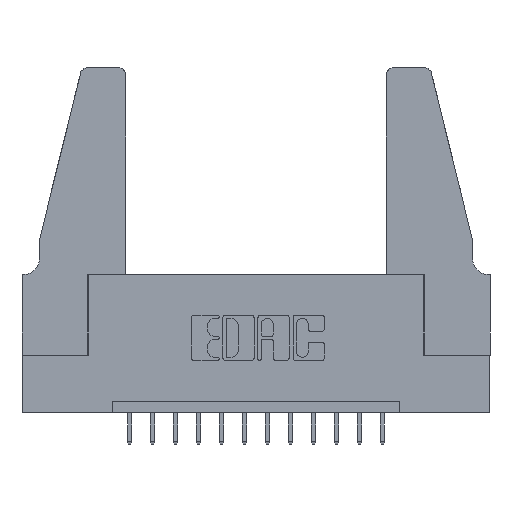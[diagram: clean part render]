
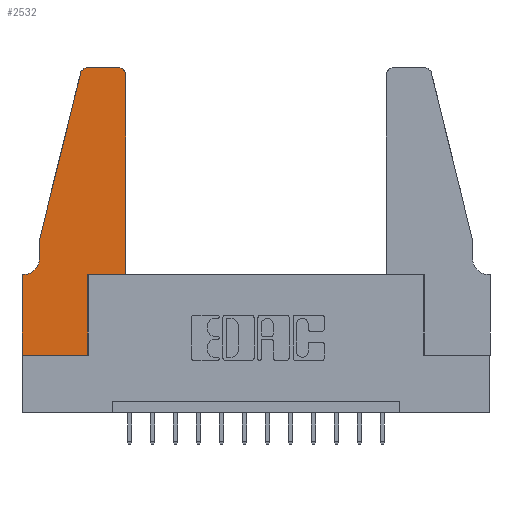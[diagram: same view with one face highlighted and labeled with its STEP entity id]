
A CAD part, top view. The second image highlights one B-rep face of the part: STEP entity #2532.
In plain terms, the highlighted planar face has unit normal (0, 0, 1).
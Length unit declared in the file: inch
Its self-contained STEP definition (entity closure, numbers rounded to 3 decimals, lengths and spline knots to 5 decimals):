
#18 = CIRCLE ( 'NONE', #11860, 0.03 ) ;
#235 = CARTESIAN_POINT ( 'NONE',  ( 0.4505, 0.35, 0.37 ) ) ;
#239 = EDGE_CURVE ( 'NONE', #14840, #13316, #10467, .T. ) ;
#318 = VERTEX_POINT ( 'NONE', #13299 ) ;
#398 = DIRECTION ( 'NONE',  ( 0., 1., 0. ) ) ;
#469 = DIRECTION ( 'NONE',  ( 0., 0., 1. ) ) ;
#522 = CARTESIAN_POINT ( 'NONE',  ( 0.0055, 0.35, 0.37 ) ) ;
#626 = VECTOR ( 'NONE', #9659, 39.37008 ) ;
#684 = CARTESIAN_POINT ( 'NONE',  ( 0.0755, 0.35, 0.37 ) ) ;
#812 = CARTESIAN_POINT ( 'NONE',  ( 0., 0., 0.37 ) ) ;
#1012 = AXIS2_PLACEMENT_3D ( 'NONE', #2104, #15271, #14018 ) ;
#1308 = PLANE ( 'NONE',  #6157 ) ;
#1349 = ORIENTED_EDGE ( 'NONE', *, *, #14159, .T. ) ;
#1703 = CARTESIAN_POINT ( 'NONE',  ( 0.4505, 0.35, 0.37 ) ) ;
#1771 = DIRECTION ( 'NONE',  ( -1., 0., 0. ) ) ;
#1816 = EDGE_CURVE ( 'NONE', #4853, #5259, #2169, .T. ) ;
#2104 = CARTESIAN_POINT ( 'NONE',  ( 0.0055, 0.42, 0.37 ) ) ;
#2169 = CIRCLE ( 'NONE', #11281, 0.03 ) ;
#2491 = DIRECTION ( 'NONE',  ( 0., -1., 0. ) ) ;
#2532 = ADVANCED_FACE ( 'NONE', ( #9259 ), #1308, .T. ) ;
#2585 = ORIENTED_EDGE ( 'NONE', *, *, #9386, .T. ) ;
#3061 = VECTOR ( 'NONE', #398, 39.37008 ) ;
#3105 = DIRECTION ( 'NONE',  ( 1., 0., 0. ) ) ;
#3205 = ORIENTED_EDGE ( 'NONE', *, *, #10355, .T. ) ;
#3351 = DIRECTION ( 'NONE',  ( -0.239, -0.971, 0. ) ) ;
#3668 = DIRECTION ( 'NONE',  ( 0., 0., 1. ) ) ;
#3844 = ORIENTED_EDGE ( 'NONE', *, *, #9119, .T. ) ;
#4301 = CARTESIAN_POINT ( 'NONE',  ( 0.4505, 0.35, 0.37 ) ) ;
#4439 = VERTEX_POINT ( 'NONE', #5909 ) ;
#4552 = ORIENTED_EDGE ( 'NONE', *, *, #239, .T. ) ;
#4595 = EDGE_CURVE ( 'NONE', #13337, #5781, #18, .T. ) ;
#4648 = DIRECTION ( 'NONE',  ( 0., 1., 0. ) ) ;
#4853 = VERTEX_POINT ( 'NONE', #13057 ) ;
#5055 = CARTESIAN_POINT ( 'NONE',  ( 0.4205, 1.25, 0.37 ) ) ;
#5165 = CARTESIAN_POINT ( 'NONE',  ( 0.2865, 0.35, 0.37 ) ) ;
#5259 = VERTEX_POINT ( 'NONE', #5055 ) ;
#5325 = CARTESIAN_POINT ( 'NONE',  ( 0.0755, 0.5, 0.37 ) ) ;
#5584 = VECTOR ( 'NONE', #2491, 39.37008 ) ;
#5622 = VECTOR ( 'NONE', #4648, 39.37008 ) ;
#5656 = ORIENTED_EDGE ( 'NONE', *, *, #6640, .T. ) ;
#5781 = VERTEX_POINT ( 'NONE', #12196 ) ;
#5879 = LINE ( 'NONE', #12349, #14713 ) ;
#5909 = CARTESIAN_POINT ( 'NONE',  ( 0.0755, 0.42, 0.37 ) ) ;
#6077 = ORIENTED_EDGE ( 'NONE', *, *, #12854, .T. ) ;
#6157 = AXIS2_PLACEMENT_3D ( 'NONE', #14259, #12823, #10567 ) ;
#6277 = VECTOR ( 'NONE', #12506, 39.37008 ) ;
#6336 = CARTESIAN_POINT ( 'NONE',  ( 0., 0., 0.37 ) ) ;
#6567 = CARTESIAN_POINT ( 'NONE',  ( 0., 0., 0.37 ) ) ;
#6640 = EDGE_CURVE ( 'NONE', #4439, #6803, #10159, .T. ) ;
#6803 = VERTEX_POINT ( 'NONE', #522 ) ;
#6937 = VERTEX_POINT ( 'NONE', #6336 ) ;
#7766 = LINE ( 'NONE', #4301, #3061 ) ;
#8425 = CARTESIAN_POINT ( 'NONE',  ( 0.284, 1.22, 0.37 ) ) ;
#8905 = DIRECTION ( 'NONE',  ( 1., 0., 0. ) ) ;
#9119 = EDGE_CURVE ( 'NONE', #6937, #14840, #10177, .T. ) ;
#9137 = VERTEX_POINT ( 'NONE', #1703 ) ;
#9193 = CARTESIAN_POINT ( 'NONE',  ( 0.0755, 0.5, 0.37 ) ) ;
#9259 = FACE_OUTER_BOUND ( 'NONE', #13640, .T. ) ;
#9386 = EDGE_CURVE ( 'NONE', #6803, #318, #14887, .T. ) ;
#9650 = DIRECTION ( 'NONE',  ( 1., 0., 0. ) ) ;
#9659 = DIRECTION ( 'NONE',  ( 1., 0., 0. ) ) ;
#9695 = VECTOR ( 'NONE', #3105, 39.37008 ) ;
#9852 = CARTESIAN_POINT ( 'NONE',  ( 0.284, 1.25, 0.37 ) ) ;
#10159 = CIRCLE ( 'NONE', #1012, 0.07 ) ;
#10177 = LINE ( 'NONE', #812, #9695 ) ;
#10355 = EDGE_CURVE ( 'NONE', #9137, #4853, #7766, .T. ) ;
#10440 = ORIENTED_EDGE ( 'NONE', *, *, #11280, .T. ) ;
#10467 = LINE ( 'NONE', #15239, #5622 ) ;
#10489 = LINE ( 'NONE', #9193, #13762 ) ;
#10567 = DIRECTION ( 'NONE',  ( 1., 0., 0. ) ) ;
#10718 = LINE ( 'NONE', #10792, #5584 ) ;
#10792 = CARTESIAN_POINT ( 'NONE',  ( 0.0755, 0.5, 0.37 ) ) ;
#10797 = LINE ( 'NONE', #235, #626 ) ;
#11254 = DIRECTION ( 'NONE',  ( 0., -1., 0. ) ) ;
#11280 = EDGE_CURVE ( 'NONE', #5259, #13337, #5879, .T. ) ;
#11281 = AXIS2_PLACEMENT_3D ( 'NONE', #12376, #469, #8905 ) ;
#11285 = VERTEX_POINT ( 'NONE', #5325 ) ;
#11482 = VECTOR ( 'NONE', #11254, 39.37008 ) ;
#11603 = ORIENTED_EDGE ( 'NONE', *, *, #4595, .T. ) ;
#11860 = AXIS2_PLACEMENT_3D ( 'NONE', #8425, #3668, #9650 ) ;
#12131 = ORIENTED_EDGE ( 'NONE', *, *, #1816, .T. ) ;
#12196 = CARTESIAN_POINT ( 'NONE',  ( 0.25487, 1.22718, 0.37 ) ) ;
#12349 = CARTESIAN_POINT ( 'NONE',  ( 0.2605, 1.25, 0.37 ) ) ;
#12376 = CARTESIAN_POINT ( 'NONE',  ( 0.4205, 1.22, 0.37 ) ) ;
#12506 = DIRECTION ( 'NONE',  ( -1., 0., 0. ) ) ;
#12778 = EDGE_CURVE ( 'NONE', #11285, #4439, #10718, .T. ) ;
#12823 = DIRECTION ( 'NONE',  ( 0., 0., 1. ) ) ;
#12854 = EDGE_CURVE ( 'NONE', #318, #6937, #13674, .T. ) ;
#13057 = CARTESIAN_POINT ( 'NONE',  ( 0.4505, 1.22, 0.37 ) ) ;
#13299 = CARTESIAN_POINT ( 'NONE',  ( 0., 0.35, 0.37 ) ) ;
#13316 = VERTEX_POINT ( 'NONE', #5165 ) ;
#13337 = VERTEX_POINT ( 'NONE', #9852 ) ;
#13506 = ORIENTED_EDGE ( 'NONE', *, *, #15125, .T. ) ;
#13640 = EDGE_LOOP ( 'NONE', ( #10440, #11603, #13506, #14587, #5656, #2585, #6077, #3844, #4552, #1349, #3205, #12131 ) ) ;
#13674 = LINE ( 'NONE', #6567, #11482 ) ;
#13762 = VECTOR ( 'NONE', #3351, 39.37008 ) ;
#14018 = DIRECTION ( 'NONE',  ( -1., 0., 0. ) ) ;
#14159 = EDGE_CURVE ( 'NONE', #13316, #9137, #10797, .T. ) ;
#14259 = CARTESIAN_POINT ( 'NONE',  ( 0., 0.35, 0.37 ) ) ;
#14369 = CARTESIAN_POINT ( 'NONE',  ( 0.2865, 0., 0.37 ) ) ;
#14587 = ORIENTED_EDGE ( 'NONE', *, *, #12778, .T. ) ;
#14713 = VECTOR ( 'NONE', #1771, 39.37008 ) ;
#14840 = VERTEX_POINT ( 'NONE', #14369 ) ;
#14887 = LINE ( 'NONE', #684, #6277 ) ;
#15125 = EDGE_CURVE ( 'NONE', #5781, #11285, #10489, .T. ) ;
#15239 = CARTESIAN_POINT ( 'NONE',  ( 0.2865, 0.35, 0.37 ) ) ;
#15271 = DIRECTION ( 'NONE',  ( 0., 0., -1. ) ) ;
